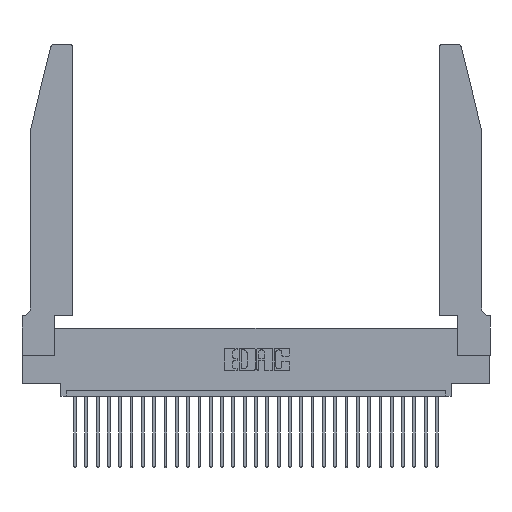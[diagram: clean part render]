
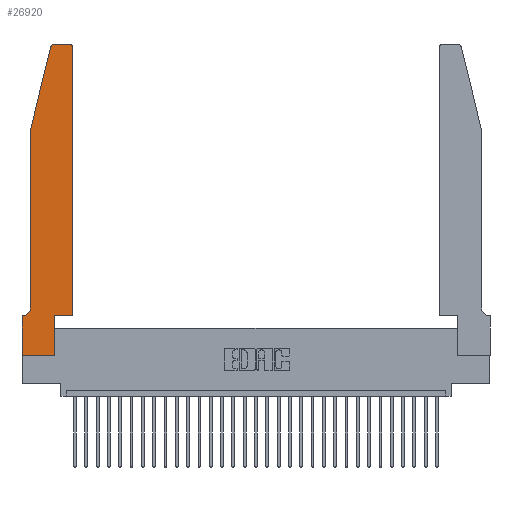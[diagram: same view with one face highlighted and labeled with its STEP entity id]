
A CAD part, top view. The second image highlights one B-rep face of the part: STEP entity #26920.
In plain terms, the highlighted planar face has unit normal (0, 0, 1).
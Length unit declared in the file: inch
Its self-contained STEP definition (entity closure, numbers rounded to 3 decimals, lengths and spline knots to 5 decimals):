
#28 = LINE ( 'NONE', #27257, #5233 ) ;
#1469 = DIRECTION ( 'NONE',  ( 0., -1., 0. ) ) ;
#1833 = VERTEX_POINT ( 'NONE', #27479 ) ;
#1890 = VECTOR ( 'NONE', #9081, 39.37008 ) ;
#2268 = CARTESIAN_POINT ( 'NONE',  ( 0.0755, 2., 0.37 ) ) ;
#2305 = CARTESIAN_POINT ( 'NONE',  ( 0.284, 2.72, 0.37 ) ) ;
#2411 = CARTESIAN_POINT ( 'NONE',  ( 0., 0., 0.37 ) ) ;
#2459 = VECTOR ( 'NONE', #18840, 39.37008 ) ;
#2892 = CARTESIAN_POINT ( 'NONE',  ( 0.0755, 0.42, 0.37 ) ) ;
#3190 = VERTEX_POINT ( 'NONE', #17188 ) ;
#3766 = EDGE_LOOP ( 'NONE', ( #15167, #11900, #18515, #8389, #4637, #17654, #27348, #20355, #8247, #17952, #4247, #5570 ) ) ;
#3963 = DIRECTION ( 'NONE',  ( 0., 1., 0. ) ) ;
#4054 = VERTEX_POINT ( 'NONE', #21752 ) ;
#4247 = ORIENTED_EDGE ( 'NONE', *, *, #27529, .T. ) ;
#4628 = CARTESIAN_POINT ( 'NONE',  ( 0.4505, 0.35, 0.37 ) ) ;
#4637 = ORIENTED_EDGE ( 'NONE', *, *, #20983, .T. ) ;
#4710 = EDGE_CURVE ( 'NONE', #27463, #28495, #25518, .T. ) ;
#4803 = LINE ( 'NONE', #9288, #11578 ) ;
#4828 = CARTESIAN_POINT ( 'NONE',  ( 0.0755, 2., 0.37 ) ) ;
#5077 = AXIS2_PLACEMENT_3D ( 'NONE', #10522, #8040, #27217 ) ;
#5233 = VECTOR ( 'NONE', #6157, 39.37008 ) ;
#5528 = VECTOR ( 'NONE', #19129, 39.37008 ) ;
#5570 = ORIENTED_EDGE ( 'NONE', *, *, #13578, .T. ) ;
#5675 = VECTOR ( 'NONE', #10727, 39.37008 ) ;
#6157 = DIRECTION ( 'NONE',  ( -1., 0., 0. ) ) ;
#7268 = CARTESIAN_POINT ( 'NONE',  ( 0.4505, 2.72, 0.37 ) ) ;
#7327 = EDGE_CURVE ( 'NONE', #11265, #29214, #25368, .T. ) ;
#7891 = EDGE_CURVE ( 'NONE', #30537, #1833, #26820, .T. ) ;
#8040 = DIRECTION ( 'NONE',  ( 0., 0., -1. ) ) ;
#8053 = CARTESIAN_POINT ( 'NONE',  ( 0., 0.35, 0.37 ) ) ;
#8247 = ORIENTED_EDGE ( 'NONE', *, *, #10279, .T. ) ;
#8389 = ORIENTED_EDGE ( 'NONE', *, *, #18397, .T. ) ;
#8447 = CARTESIAN_POINT ( 'NONE',  ( 0.4205, 2.72, 0.37 ) ) ;
#8540 = LINE ( 'NONE', #27867, #18259 ) ;
#9081 = DIRECTION ( 'NONE',  ( 0., -1., 0. ) ) ;
#9122 = CARTESIAN_POINT ( 'NONE',  ( 0.25487, 2.72718, 0.37 ) ) ;
#9248 = AXIS2_PLACEMENT_3D ( 'NONE', #8053, #17862, #20290 ) ;
#9273 = DIRECTION ( 'NONE',  ( 0., 0., 1. ) ) ;
#9288 = CARTESIAN_POINT ( 'NONE',  ( 0.2865, 0.35, 0.37 ) ) ;
#9317 = EDGE_CURVE ( 'NONE', #4054, #28278, #24127, .T. ) ;
#10053 = FACE_OUTER_BOUND ( 'NONE', #3766, .T. ) ;
#10279 = EDGE_CURVE ( 'NONE', #29214, #4054, #4803, .T. ) ;
#10316 = VERTEX_POINT ( 'NONE', #2892 ) ;
#10522 = CARTESIAN_POINT ( 'NONE',  ( 0.0055, 0.42, 0.37 ) ) ;
#10727 = DIRECTION ( 'NONE',  ( -0.239, -0.971, 0. ) ) ;
#11188 = AXIS2_PLACEMENT_3D ( 'NONE', #8447, #9273, #18984 ) ;
#11265 = VERTEX_POINT ( 'NONE', #23161 ) ;
#11578 = VECTOR ( 'NONE', #21948, 39.37008 ) ;
#11900 = ORIENTED_EDGE ( 'NONE', *, *, #25072, .T. ) ;
#12731 = PLANE ( 'NONE',  #9248 ) ;
#13097 = CIRCLE ( 'NONE', #23600, 0.03 ) ;
#13578 = EDGE_CURVE ( 'NONE', #30792, #14943, #24853, .T. ) ;
#13996 = DIRECTION ( 'NONE',  ( -1., 0., 0. ) ) ;
#14943 = VERTEX_POINT ( 'NONE', #28580 ) ;
#15167 = ORIENTED_EDGE ( 'NONE', *, *, #25676, .T. ) ;
#15764 = CARTESIAN_POINT ( 'NONE',  ( 0.0055, 0.35, 0.37 ) ) ;
#17188 = CARTESIAN_POINT ( 'NONE',  ( 0.284, 2.75, 0.37 ) ) ;
#17654 = ORIENTED_EDGE ( 'NONE', *, *, #7891, .T. ) ;
#17845 = VECTOR ( 'NONE', #13996, 39.37008 ) ;
#17862 = DIRECTION ( 'NONE',  ( 0., 0., 1. ) ) ;
#17952 = ORIENTED_EDGE ( 'NONE', *, *, #9317, .T. ) ;
#18156 = CARTESIAN_POINT ( 'NONE',  ( 0.0755, 2., 0.37 ) ) ;
#18259 = VECTOR ( 'NONE', #3963, 39.37008 ) ;
#18397 = EDGE_CURVE ( 'NONE', #28495, #10316, #19856, .T. ) ;
#18515 = ORIENTED_EDGE ( 'NONE', *, *, #4710, .T. ) ;
#18700 = CARTESIAN_POINT ( 'NONE',  ( 0.0755, 0.35, 0.37 ) ) ;
#18840 = DIRECTION ( 'NONE',  ( 1., 0., 0. ) ) ;
#18984 = DIRECTION ( 'NONE',  ( 1., 0., 0. ) ) ;
#19129 = DIRECTION ( 'NONE',  ( 1., 0., 0. ) ) ;
#19856 = LINE ( 'NONE', #2268, #1890 ) ;
#20290 = DIRECTION ( 'NONE',  ( 1., 0., 0. ) ) ;
#20355 = ORIENTED_EDGE ( 'NONE', *, *, #7327, .T. ) ;
#20983 = EDGE_CURVE ( 'NONE', #10316, #30537, #30134, .T. ) ;
#21752 = CARTESIAN_POINT ( 'NONE',  ( 0.2865, 0.35, 0.37 ) ) ;
#21948 = DIRECTION ( 'NONE',  ( 0., 1., 0. ) ) ;
#22024 = EDGE_CURVE ( 'NONE', #1833, #11265, #29348, .T. ) ;
#23161 = CARTESIAN_POINT ( 'NONE',  ( 0., 0., 0.37 ) ) ;
#23544 = CARTESIAN_POINT ( 'NONE',  ( 0.4505, 0.35, 0.37 ) ) ;
#23600 = AXIS2_PLACEMENT_3D ( 'NONE', #2305, #28389, #28603 ) ;
#24127 = LINE ( 'NONE', #23544, #2459 ) ;
#24253 = CARTESIAN_POINT ( 'NONE',  ( 0.2865, 0., 0.37 ) ) ;
#24853 = CIRCLE ( 'NONE', #11188, 0.03 ) ;
#25072 = EDGE_CURVE ( 'NONE', #3190, #27463, #13097, .T. ) ;
#25368 = LINE ( 'NONE', #2411, #5528 ) ;
#25518 = LINE ( 'NONE', #18156, #5675 ) ;
#25676 = EDGE_CURVE ( 'NONE', #14943, #3190, #28, .T. ) ;
#26820 = LINE ( 'NONE', #18700, #17845 ) ;
#26920 = ADVANCED_FACE ( 'NONE', ( #10053 ), #12731, .T. ) ;
#27217 = DIRECTION ( 'NONE',  ( -1., 0., 0. ) ) ;
#27257 = CARTESIAN_POINT ( 'NONE',  ( 0.2605, 2.75, 0.37 ) ) ;
#27348 = ORIENTED_EDGE ( 'NONE', *, *, #22024, .T. ) ;
#27463 = VERTEX_POINT ( 'NONE', #9122 ) ;
#27479 = CARTESIAN_POINT ( 'NONE',  ( 0., 0.35, 0.37 ) ) ;
#27484 = VECTOR ( 'NONE', #1469, 39.37008 ) ;
#27529 = EDGE_CURVE ( 'NONE', #28278, #30792, #8540, .T. ) ;
#27867 = CARTESIAN_POINT ( 'NONE',  ( 0.4505, 0.35, 0.37 ) ) ;
#28278 = VERTEX_POINT ( 'NONE', #4628 ) ;
#28389 = DIRECTION ( 'NONE',  ( 0., 0., 1. ) ) ;
#28495 = VERTEX_POINT ( 'NONE', #4828 ) ;
#28580 = CARTESIAN_POINT ( 'NONE',  ( 0.4205, 2.75, 0.37 ) ) ;
#28603 = DIRECTION ( 'NONE',  ( 1., 0., 0. ) ) ;
#29214 = VERTEX_POINT ( 'NONE', #24253 ) ;
#29348 = LINE ( 'NONE', #30307, #27484 ) ;
#30134 = CIRCLE ( 'NONE', #5077, 0.07 ) ;
#30307 = CARTESIAN_POINT ( 'NONE',  ( 0., 0., 0.37 ) ) ;
#30537 = VERTEX_POINT ( 'NONE', #15764 ) ;
#30792 = VERTEX_POINT ( 'NONE', #7268 ) ;
